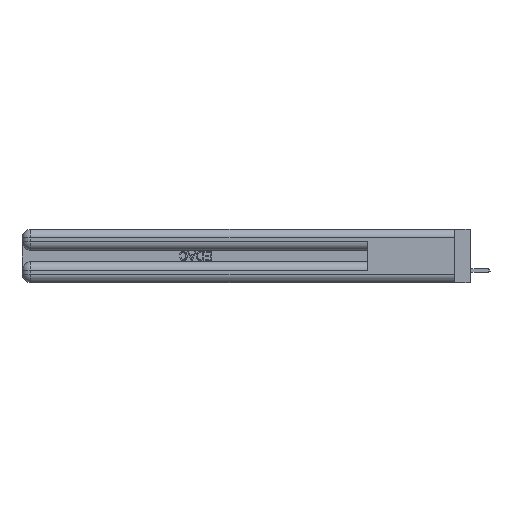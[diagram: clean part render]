
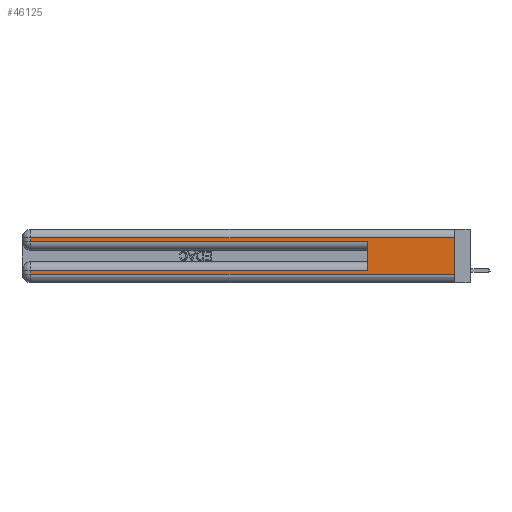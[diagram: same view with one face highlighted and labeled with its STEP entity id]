
A CAD part, left-side view. The second image highlights one B-rep face of the part: STEP entity #46125.
In plain terms, the highlighted planar face has unit normal (-1, 0, 0).
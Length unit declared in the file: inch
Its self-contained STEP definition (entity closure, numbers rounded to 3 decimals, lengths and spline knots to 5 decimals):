
#56 = VERTEX_POINT ( 'NONE', #38696 ) ;
#261 = ORIENTED_EDGE ( 'NONE', *, *, #2797, .T. ) ;
#578 = LINE ( 'NONE', #10782, #15150 ) ;
#1534 = VERTEX_POINT ( 'NONE', #24602 ) ;
#1953 = VERTEX_POINT ( 'NONE', #16658 ) ;
#2547 = CARTESIAN_POINT ( 'NONE',  ( 0., 2.94, 0.085 ) ) ;
#2797 = EDGE_CURVE ( 'NONE', #20047, #20845, #8011, .T. ) ;
#2853 = ORIENTED_EDGE ( 'NONE', *, *, #21345, .T. ) ;
#2878 = VERTEX_POINT ( 'NONE', #15439 ) ;
#2954 = VECTOR ( 'NONE', #28732, 39.37008 ) ;
#3147 = VERTEX_POINT ( 'NONE', #53832 ) ;
#5651 = EDGE_CURVE ( 'NONE', #3147, #56, #38312, .T. ) ;
#6483 = CARTESIAN_POINT ( 'NONE',  ( 0., 2.94, 0.37 ) ) ;
#8011 = LINE ( 'NONE', #26381, #45236 ) ;
#9240 = DIRECTION ( 'NONE',  ( 0., 0., -1. ) ) ;
#10782 = CARTESIAN_POINT ( 'NONE',  ( 0., 0.6, 0.145 ) ) ;
#11615 = DIRECTION ( 'NONE',  ( 0., -1., 0. ) ) ;
#12527 = ORIENTED_EDGE ( 'NONE', *, *, #5651, .T. ) ;
#12667 = VECTOR ( 'NONE', #11615, 39.37008 ) ;
#12935 = CARTESIAN_POINT ( 'NONE',  ( 0., 0., 0.37 ) ) ;
#15150 = VECTOR ( 'NONE', #27452, 39.37008 ) ;
#15439 = CARTESIAN_POINT ( 'NONE',  ( 0., 0.6, 0.085 ) ) ;
#15708 = CARTESIAN_POINT ( 'NONE',  ( 0., 0., 0.06 ) ) ;
#16523 = CARTESIAN_POINT ( 'NONE',  ( 0., 0., 0.37 ) ) ;
#16658 = CARTESIAN_POINT ( 'NONE',  ( 0., 0.6, 0.285 ) ) ;
#17454 = DIRECTION ( 'NONE',  ( 1., 0., 0. ) ) ;
#17629 = VECTOR ( 'NONE', #25140, 39.37008 ) ;
#17763 = EDGE_CURVE ( 'NONE', #1534, #1953, #25146, .T. ) ;
#18480 = VECTOR ( 'NONE', #49088, 39.37008 ) ;
#18659 = DIRECTION ( 'NONE',  ( 0., 0., -1. ) ) ;
#20047 = VERTEX_POINT ( 'NONE', #43321 ) ;
#20845 = VERTEX_POINT ( 'NONE', #42942 ) ;
#21220 = EDGE_LOOP ( 'NONE', ( #50599, #261, #49566, #31542, #42000, #2853, #42388, #12527 ) ) ;
#21345 = EDGE_CURVE ( 'NONE', #2878, #54196, #23791, .T. ) ;
#22682 = DIRECTION ( 'NONE',  ( 0., 1., 0. ) ) ;
#23791 = LINE ( 'NONE', #47693, #36250 ) ;
#24602 = CARTESIAN_POINT ( 'NONE',  ( 0., 2.94, 0.285 ) ) ;
#25140 = DIRECTION ( 'NONE',  ( 0., 0., -1. ) ) ;
#25146 = LINE ( 'NONE', #36695, #12667 ) ;
#26381 = CARTESIAN_POINT ( 'NONE',  ( 0., 0., 0.31 ) ) ;
#26942 = CARTESIAN_POINT ( 'NONE',  ( 0., 2.94, 0.37 ) ) ;
#27452 = DIRECTION ( 'NONE',  ( 0., 0., 1. ) ) ;
#28732 = DIRECTION ( 'NONE',  ( 0., -1., 0. ) ) ;
#31542 = ORIENTED_EDGE ( 'NONE', *, *, #17763, .T. ) ;
#33991 = VECTOR ( 'NONE', #18659, 39.37008 ) ;
#35439 = EDGE_CURVE ( 'NONE', #54196, #3147, #45075, .T. ) ;
#36015 = LINE ( 'NONE', #16523, #17629 ) ;
#36250 = VECTOR ( 'NONE', #22682, 39.37008 ) ;
#36695 = CARTESIAN_POINT ( 'NONE',  ( 0., 0., 0.285 ) ) ;
#38312 = LINE ( 'NONE', #15708, #2954 ) ;
#38696 = CARTESIAN_POINT ( 'NONE',  ( 0., 0., 0.06 ) ) ;
#39832 = EDGE_CURVE ( 'NONE', #20845, #1534, #45351, .T. ) ;
#40863 = EDGE_CURVE ( 'NONE', #2878, #1953, #578, .T. ) ;
#41676 = AXIS2_PLACEMENT_3D ( 'NONE', #12935, #17454, #9240 ) ;
#42000 = ORIENTED_EDGE ( 'NONE', *, *, #40863, .F. ) ;
#42388 = ORIENTED_EDGE ( 'NONE', *, *, #35439, .T. ) ;
#42942 = CARTESIAN_POINT ( 'NONE',  ( 0., 2.94, 0.31 ) ) ;
#43134 = DIRECTION ( 'NONE',  ( 0., 1., 0. ) ) ;
#43321 = CARTESIAN_POINT ( 'NONE',  ( 0., 0., 0.31 ) ) ;
#45075 = LINE ( 'NONE', #26942, #33991 ) ;
#45236 = VECTOR ( 'NONE', #43134, 39.37008 ) ;
#45351 = LINE ( 'NONE', #6483, #18480 ) ;
#46125 = ADVANCED_FACE ( 'NONE', ( #46230 ), #50685, .F. ) ;
#46230 = FACE_OUTER_BOUND ( 'NONE', #21220, .T. ) ;
#47693 = CARTESIAN_POINT ( 'NONE',  ( 0., 0., 0.085 ) ) ;
#49088 = DIRECTION ( 'NONE',  ( 0., 0., -1. ) ) ;
#49566 = ORIENTED_EDGE ( 'NONE', *, *, #39832, .T. ) ;
#50159 = EDGE_CURVE ( 'NONE', #20047, #56, #36015, .T. ) ;
#50599 = ORIENTED_EDGE ( 'NONE', *, *, #50159, .F. ) ;
#50685 = PLANE ( 'NONE',  #41676 ) ;
#53832 = CARTESIAN_POINT ( 'NONE',  ( 0., 2.94, 0.06 ) ) ;
#54196 = VERTEX_POINT ( 'NONE', #2547 ) ;
